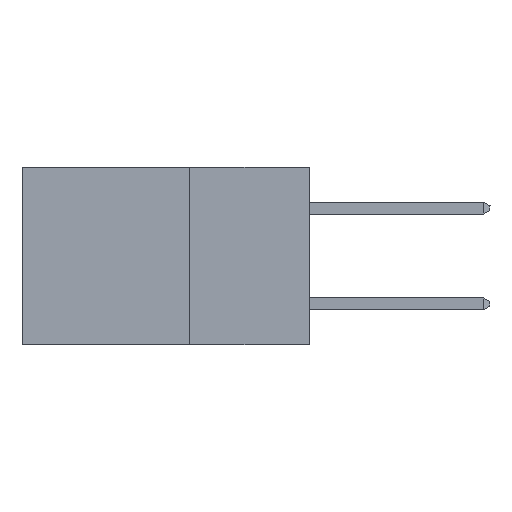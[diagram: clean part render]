
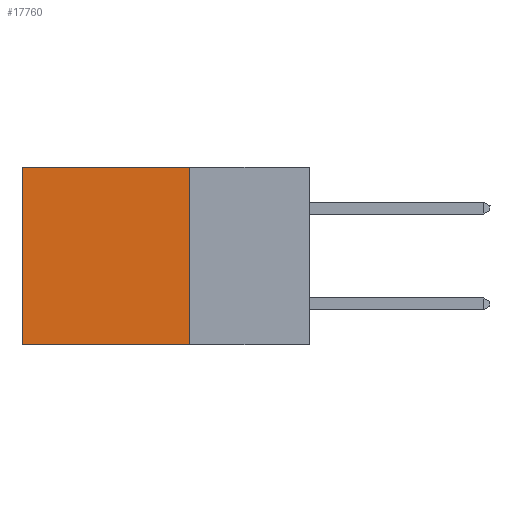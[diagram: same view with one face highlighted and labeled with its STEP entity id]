
A CAD part, left-side view. The second image highlights one B-rep face of the part: STEP entity #17760.
In plain terms, the highlighted planar face has unit normal (-1, 0, 0).
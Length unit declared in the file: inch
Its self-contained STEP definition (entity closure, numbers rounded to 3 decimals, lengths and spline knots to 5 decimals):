
#989 = VECTOR ( 'NONE', #12597, 39.37008 ) ;
#1143 = LINE ( 'NONE', #8984, #989 ) ;
#1903 = VERTEX_POINT ( 'NONE', #34139 ) ;
#2582 = EDGE_CURVE ( 'NONE', #41692, #1903, #19631, .T. ) ;
#3378 = DIRECTION ( 'NONE',  ( 0., 0., -1. ) ) ;
#4348 = PLANE ( 'NONE',  #16587 ) ;
#8056 = DIRECTION ( 'NONE',  ( 1., 0., 0. ) ) ;
#8984 = CARTESIAN_POINT ( 'NONE',  ( 0.2875, 0.25, 0. ) ) ;
#12597 = DIRECTION ( 'NONE',  ( 0., 0., -1. ) ) ;
#12786 = ORIENTED_EDGE ( 'NONE', *, *, #17580, .T. ) ;
#12888 = CARTESIAN_POINT ( 'NONE',  ( 0.2875, 0.25, 0. ) ) ;
#13410 = CARTESIAN_POINT ( 'NONE',  ( 0.2875, 0.25, 0. ) ) ;
#14252 = CARTESIAN_POINT ( 'NONE',  ( 0.2875, 0.25, -0.37 ) ) ;
#14545 = EDGE_CURVE ( 'NONE', #26697, #30868, #21987, .T. ) ;
#16571 = DIRECTION ( 'NONE',  ( 0., 1., 0. ) ) ;
#16587 = AXIS2_PLACEMENT_3D ( 'NONE', #42782, #8056, #32877 ) ;
#17021 = DIRECTION ( 'NONE',  ( 0., 1., 0. ) ) ;
#17149 = ORIENTED_EDGE ( 'NONE', *, *, #39267, .F. ) ;
#17580 = EDGE_CURVE ( 'NONE', #1903, #30868, #36694, .T. ) ;
#17760 = ADVANCED_FACE ( 'NONE', ( #39520 ), #4348, .F. ) ;
#19500 = VECTOR ( 'NONE', #17021, 39.37008 ) ;
#19631 = LINE ( 'NONE', #13410, #19500 ) ;
#21897 = VECTOR ( 'NONE', #16571, 39.37008 ) ;
#21987 = LINE ( 'NONE', #34124, #21897 ) ;
#24905 = EDGE_LOOP ( 'NONE', ( #12786, #25597, #17149, #37381 ) ) ;
#25597 = ORIENTED_EDGE ( 'NONE', *, *, #14545, .F. ) ;
#26697 = VERTEX_POINT ( 'NONE', #14252 ) ;
#30868 = VERTEX_POINT ( 'NONE', #42128 ) ;
#32877 = DIRECTION ( 'NONE',  ( 0., 0., -1. ) ) ;
#34124 = CARTESIAN_POINT ( 'NONE',  ( 0.2875, 0.25, -0.37 ) ) ;
#34139 = CARTESIAN_POINT ( 'NONE',  ( 0.2875, 0.6, 0. ) ) ;
#35273 = CARTESIAN_POINT ( 'NONE',  ( 0.2875, 0.6, 0. ) ) ;
#36694 = LINE ( 'NONE', #35273, #37699 ) ;
#37381 = ORIENTED_EDGE ( 'NONE', *, *, #2582, .T. ) ;
#37699 = VECTOR ( 'NONE', #3378, 39.37008 ) ;
#39267 = EDGE_CURVE ( 'NONE', #41692, #26697, #1143, .T. ) ;
#39520 = FACE_OUTER_BOUND ( 'NONE', #24905, .T. ) ;
#41692 = VERTEX_POINT ( 'NONE', #12888 ) ;
#42128 = CARTESIAN_POINT ( 'NONE',  ( 0.2875, 0.6, -0.37 ) ) ;
#42782 = CARTESIAN_POINT ( 'NONE',  ( 0.2875, 0.25, 0. ) ) ;
